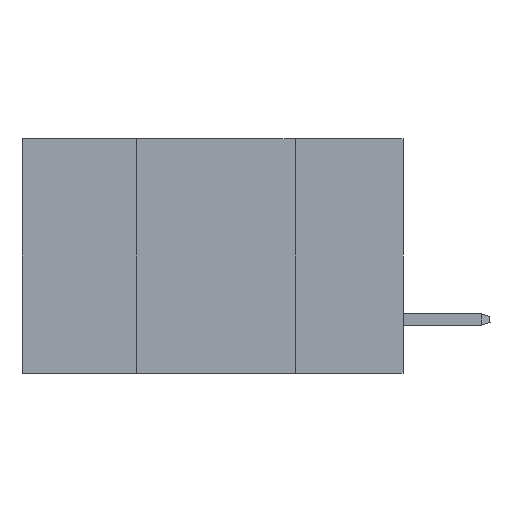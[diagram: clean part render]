
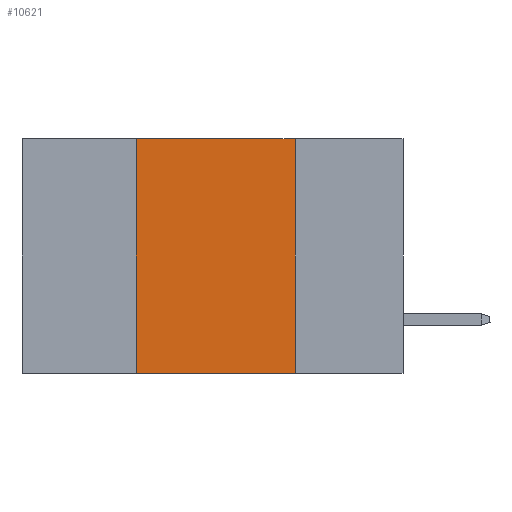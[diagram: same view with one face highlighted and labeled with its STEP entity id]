
A CAD part, left-side view. The second image highlights one B-rep face of the part: STEP entity #10621.
In plain terms, the highlighted planar face has unit normal (-1, 0, 0).
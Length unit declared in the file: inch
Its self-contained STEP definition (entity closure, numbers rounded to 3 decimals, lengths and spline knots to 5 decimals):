
#1063 = CARTESIAN_POINT ( 'NONE',  ( 0., 0.6, 0. ) ) ;
#1340 = CARTESIAN_POINT ( 'NONE',  ( 0., 0.17, 0. ) ) ;
#2277 = VERTEX_POINT ( 'NONE', #16456 ) ;
#2616 = CARTESIAN_POINT ( 'NONE',  ( 0., 0.42, -0.37 ) ) ;
#2799 = LINE ( 'NONE', #8906, #21007 ) ;
#3239 = PLANE ( 'NONE',  #10984 ) ;
#4729 = CARTESIAN_POINT ( 'NONE',  ( 0., 0.42, 0. ) ) ;
#5279 = LINE ( 'NONE', #14112, #15131 ) ;
#5784 = DIRECTION ( 'NONE',  ( 0., 0., -1. ) ) ;
#7580 = CARTESIAN_POINT ( 'NONE',  ( 0., 0.17, -0.37 ) ) ;
#7648 = CARTESIAN_POINT ( 'NONE',  ( 0., 0.17, 0. ) ) ;
#8906 = CARTESIAN_POINT ( 'NONE',  ( 0., 0.6, -0.37 ) ) ;
#10578 = ORIENTED_EDGE ( 'NONE', *, *, #12296, .F. ) ;
#10621 = ADVANCED_FACE ( 'NONE', ( #12380 ), #3239, .F. ) ;
#10984 = AXIS2_PLACEMENT_3D ( 'NONE', #1063, #16748, #16447 ) ;
#12296 = EDGE_CURVE ( 'NONE', #2277, #18211, #5279, .T. ) ;
#12380 = FACE_OUTER_BOUND ( 'NONE', #25486, .T. ) ;
#13862 = LINE ( 'NONE', #4729, #21524 ) ;
#13994 = ORIENTED_EDGE ( 'NONE', *, *, #24531, .T. ) ;
#14112 = CARTESIAN_POINT ( 'NONE',  ( 0., 0.6, 0. ) ) ;
#15131 = VECTOR ( 'NONE', #22988, 39.37008 ) ;
#16144 = ORIENTED_EDGE ( 'NONE', *, *, #20305, .F. ) ;
#16447 = DIRECTION ( 'NONE',  ( 0., 0., -1. ) ) ;
#16456 = CARTESIAN_POINT ( 'NONE',  ( 0., 0.42, 0. ) ) ;
#16748 = DIRECTION ( 'NONE',  ( 1., 0., 0. ) ) ;
#17289 = VECTOR ( 'NONE', #5784, 39.37008 ) ;
#18211 = VERTEX_POINT ( 'NONE', #1340 ) ;
#18828 = LINE ( 'NONE', #7648, #17289 ) ;
#20305 = EDGE_CURVE ( 'NONE', #18211, #20538, #18828, .T. ) ;
#20538 = VERTEX_POINT ( 'NONE', #7580 ) ;
#21007 = VECTOR ( 'NONE', #24581, 39.37008 ) ;
#21524 = VECTOR ( 'NONE', #26950, 39.37008 ) ;
#22988 = DIRECTION ( 'NONE',  ( 0., -1., 0. ) ) ;
#24531 = EDGE_CURVE ( 'NONE', #26279, #20538, #2799, .T. ) ;
#24581 = DIRECTION ( 'NONE',  ( 0., -1., 0. ) ) ;
#24767 = ORIENTED_EDGE ( 'NONE', *, *, #27091, .F. ) ;
#25486 = EDGE_LOOP ( 'NONE', ( #16144, #10578, #24767, #13994 ) ) ;
#26279 = VERTEX_POINT ( 'NONE', #2616 ) ;
#26950 = DIRECTION ( 'NONE',  ( 0., 0., 1. ) ) ;
#27091 = EDGE_CURVE ( 'NONE', #26279, #2277, #13862, .T. ) ;
